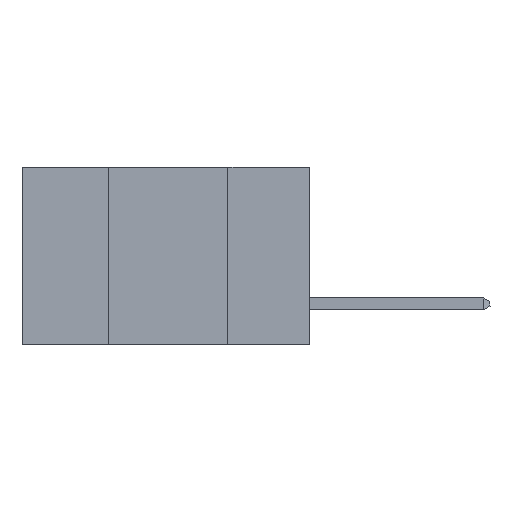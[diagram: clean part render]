
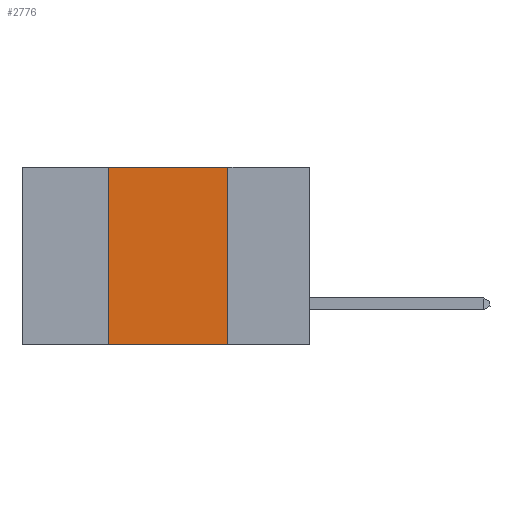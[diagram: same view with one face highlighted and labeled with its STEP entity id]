
A CAD part, left-side view. The second image highlights one B-rep face of the part: STEP entity #2776.
In plain terms, the highlighted planar face has unit normal (-1, 0, 0).
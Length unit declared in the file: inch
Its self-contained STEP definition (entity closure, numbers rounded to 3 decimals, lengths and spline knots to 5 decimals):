
#512 = VERTEX_POINT ( 'NONE', #8090 ) ;
#547 = FACE_OUTER_BOUND ( 'NONE', #18921, .T. ) ;
#1419 = CARTESIAN_POINT ( 'NONE',  ( 0., 0.6, 0. ) ) ;
#1619 = CARTESIAN_POINT ( 'NONE',  ( 0., 0.17, -0.37 ) ) ;
#2408 = VECTOR ( 'NONE', #19573, 39.37008 ) ;
#2776 = ADVANCED_FACE ( 'NONE', ( #547 ), #10946, .F. ) ;
#3011 = DIRECTION ( 'NONE',  ( 1., 0., 0. ) ) ;
#3618 = CARTESIAN_POINT ( 'NONE',  ( 0., 0.42, 0. ) ) ;
#4662 = ORIENTED_EDGE ( 'NONE', *, *, #9259, .T. ) ;
#4861 = VECTOR ( 'NONE', #17660, 39.37008 ) ;
#5188 = LINE ( 'NONE', #10552, #17449 ) ;
#5204 = DIRECTION ( 'NONE',  ( 0., 0., 1. ) ) ;
#6645 = AXIS2_PLACEMENT_3D ( 'NONE', #1419, #3011, #14147 ) ;
#7086 = EDGE_CURVE ( 'NONE', #512, #12302, #16288, .T. ) ;
#8090 = CARTESIAN_POINT ( 'NONE',  ( 0., 0.42, -0.37 ) ) ;
#8284 = ORIENTED_EDGE ( 'NONE', *, *, #17466, .F. ) ;
#9259 = EDGE_CURVE ( 'NONE', #512, #16020, #5188, .T. ) ;
#9340 = CARTESIAN_POINT ( 'NONE',  ( 0., 0.42, 0. ) ) ;
#9554 = ORIENTED_EDGE ( 'NONE', *, *, #7086, .F. ) ;
#10552 = CARTESIAN_POINT ( 'NONE',  ( 0., 0.6, -0.37 ) ) ;
#10946 = PLANE ( 'NONE',  #6645 ) ;
#12144 = DIRECTION ( 'NONE',  ( 0., -1., 0. ) ) ;
#12302 = VERTEX_POINT ( 'NONE', #9340 ) ;
#12343 = LINE ( 'NONE', #16046, #4861 ) ;
#12442 = VERTEX_POINT ( 'NONE', #17716 ) ;
#14147 = DIRECTION ( 'NONE',  ( 0., 0., -1. ) ) ;
#14861 = CARTESIAN_POINT ( 'NONE',  ( 0., 0.6, 0. ) ) ;
#15627 = LINE ( 'NONE', #14861, #2408 ) ;
#15799 = VECTOR ( 'NONE', #5204, 39.37008 ) ;
#16020 = VERTEX_POINT ( 'NONE', #1619 ) ;
#16046 = CARTESIAN_POINT ( 'NONE',  ( 0., 0.17, 0. ) ) ;
#16288 = LINE ( 'NONE', #3618, #15799 ) ;
#16807 = ORIENTED_EDGE ( 'NONE', *, *, #17788, .F. ) ;
#17449 = VECTOR ( 'NONE', #12144, 39.37008 ) ;
#17466 = EDGE_CURVE ( 'NONE', #12302, #12442, #15627, .T. ) ;
#17660 = DIRECTION ( 'NONE',  ( 0., 0., -1. ) ) ;
#17716 = CARTESIAN_POINT ( 'NONE',  ( 0., 0.17, 0. ) ) ;
#17788 = EDGE_CURVE ( 'NONE', #12442, #16020, #12343, .T. ) ;
#18921 = EDGE_LOOP ( 'NONE', ( #16807, #8284, #9554, #4662 ) ) ;
#19573 = DIRECTION ( 'NONE',  ( 0., -1., 0. ) ) ;
